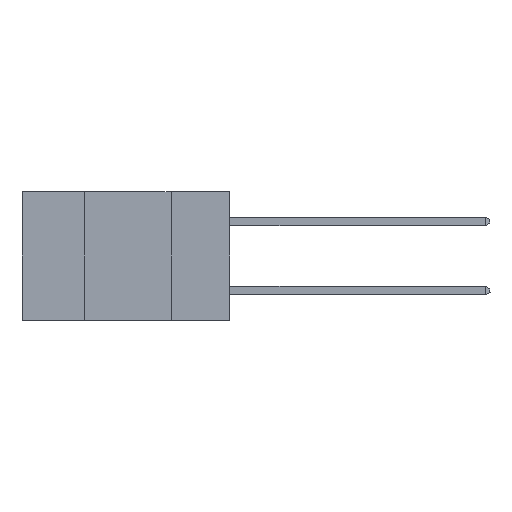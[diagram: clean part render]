
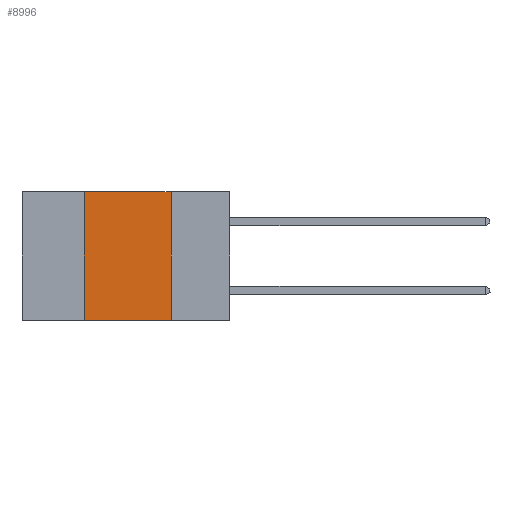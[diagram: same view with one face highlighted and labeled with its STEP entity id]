
A CAD part, left-side view. The second image highlights one B-rep face of the part: STEP entity #8996.
In plain terms, the highlighted planar face has unit normal (-1, 0, 0).
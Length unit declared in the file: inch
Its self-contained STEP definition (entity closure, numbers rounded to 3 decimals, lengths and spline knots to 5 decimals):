
#499 = ORIENTED_EDGE ( 'NONE', *, *, #6187, .T. ) ;
#1616 = CARTESIAN_POINT ( 'NONE',  ( 0., 0.17, 0. ) ) ;
#1799 = CARTESIAN_POINT ( 'NONE',  ( 0., 0.6, 0. ) ) ;
#1902 = VECTOR ( 'NONE', #7760, 39.37008 ) ;
#2387 = CARTESIAN_POINT ( 'NONE',  ( 0., 0.42, 0. ) ) ;
#3467 = DIRECTION ( 'NONE',  ( 0., 0., 1. ) ) ;
#3968 = EDGE_CURVE ( 'NONE', #14686, #12618, #5111, .T. ) ;
#4314 = VERTEX_POINT ( 'NONE', #8156 ) ;
#5111 = LINE ( 'NONE', #1799, #1902 ) ;
#5595 = ORIENTED_EDGE ( 'NONE', *, *, #11556, .F. ) ;
#5606 = LINE ( 'NONE', #9181, #11611 ) ;
#5730 = CARTESIAN_POINT ( 'NONE',  ( 0., 0.17, -0.37 ) ) ;
#5807 = CARTESIAN_POINT ( 'NONE',  ( 0., 0.42, 0. ) ) ;
#6187 = EDGE_CURVE ( 'NONE', #4314, #8496, #14083, .T. ) ;
#6630 = LINE ( 'NONE', #5807, #6995 ) ;
#6995 = VECTOR ( 'NONE', #3467, 39.37008 ) ;
#7657 = EDGE_CURVE ( 'NONE', #12618, #8496, #5606, .T. ) ;
#7760 = DIRECTION ( 'NONE',  ( 0., -1., 0. ) ) ;
#7783 = DIRECTION ( 'NONE',  ( 0., 0., -1. ) ) ;
#8156 = CARTESIAN_POINT ( 'NONE',  ( 0., 0.42, -0.37 ) ) ;
#8496 = VERTEX_POINT ( 'NONE', #5730 ) ;
#8931 = CARTESIAN_POINT ( 'NONE',  ( 0., 0.6, -0.37 ) ) ;
#8996 = ADVANCED_FACE ( 'NONE', ( #13445 ), #11410, .F. ) ;
#9159 = CARTESIAN_POINT ( 'NONE',  ( 0., 0.6, 0. ) ) ;
#9181 = CARTESIAN_POINT ( 'NONE',  ( 0., 0.17, 0. ) ) ;
#9615 = ORIENTED_EDGE ( 'NONE', *, *, #7657, .F. ) ;
#10138 = EDGE_LOOP ( 'NONE', ( #9615, #14119, #5595, #499 ) ) ;
#10359 = DIRECTION ( 'NONE',  ( 1., 0., 0. ) ) ;
#10864 = VECTOR ( 'NONE', #12650, 39.37008 ) ;
#11410 = PLANE ( 'NONE',  #13594 ) ;
#11556 = EDGE_CURVE ( 'NONE', #4314, #14686, #6630, .T. ) ;
#11611 = VECTOR ( 'NONE', #11637, 39.37008 ) ;
#11637 = DIRECTION ( 'NONE',  ( 0., 0., -1. ) ) ;
#12618 = VERTEX_POINT ( 'NONE', #1616 ) ;
#12650 = DIRECTION ( 'NONE',  ( 0., -1., 0. ) ) ;
#13445 = FACE_OUTER_BOUND ( 'NONE', #10138, .T. ) ;
#13594 = AXIS2_PLACEMENT_3D ( 'NONE', #9159, #10359, #7783 ) ;
#14083 = LINE ( 'NONE', #8931, #10864 ) ;
#14119 = ORIENTED_EDGE ( 'NONE', *, *, #3968, .F. ) ;
#14686 = VERTEX_POINT ( 'NONE', #2387 ) ;
